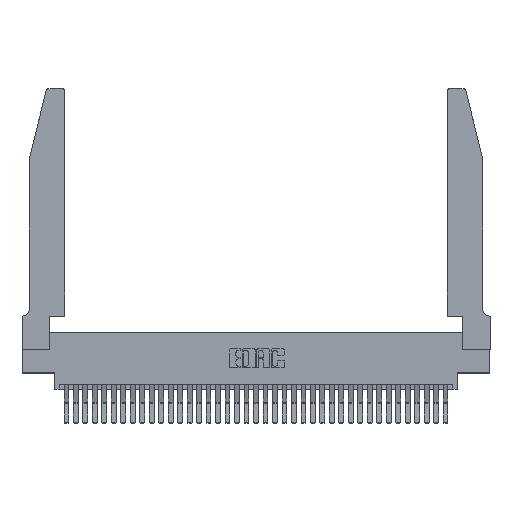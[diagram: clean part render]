
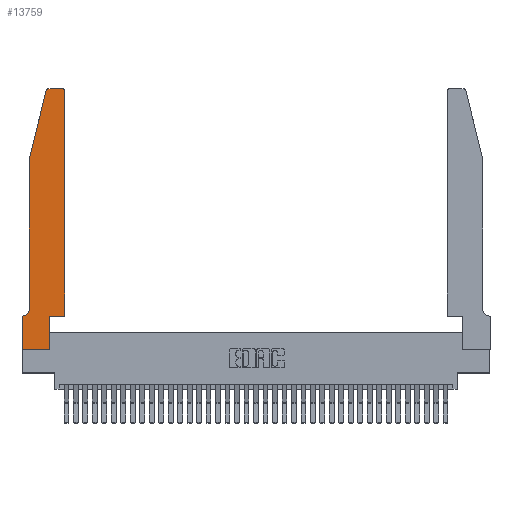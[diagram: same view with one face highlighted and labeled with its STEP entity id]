
A CAD part, top view. The second image highlights one B-rep face of the part: STEP entity #13759.
In plain terms, the highlighted planar face has unit normal (0, 0, 1).
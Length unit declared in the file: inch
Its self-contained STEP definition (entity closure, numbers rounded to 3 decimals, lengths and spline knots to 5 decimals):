
#987 = VERTEX_POINT ( 'NONE', #4956 ) ;
#1030 = EDGE_CURVE ( 'NONE', #20445, #4806, #24378, .T. ) ;
#1146 = DIRECTION ( 'NONE',  ( 0., 1., 0. ) ) ;
#1535 = ORIENTED_EDGE ( 'NONE', *, *, #20701, .T. ) ;
#1690 = CARTESIAN_POINT ( 'NONE',  ( 0.4505, 0.35, 0.37 ) ) ;
#2357 = ORIENTED_EDGE ( 'NONE', *, *, #13382, .T. ) ;
#2497 = CARTESIAN_POINT ( 'NONE',  ( 0.0755, 2., 0.37 ) ) ;
#2549 = CIRCLE ( 'NONE', #15674, 0.03 ) ;
#2687 = VERTEX_POINT ( 'NONE', #11166 ) ;
#3035 = VECTOR ( 'NONE', #26420, 39.37008 ) ;
#3300 = CARTESIAN_POINT ( 'NONE',  ( 0.0055, 0.35, 0.37 ) ) ;
#4227 = ORIENTED_EDGE ( 'NONE', *, *, #7650, .T. ) ;
#4806 = VERTEX_POINT ( 'NONE', #6256 ) ;
#4956 = CARTESIAN_POINT ( 'NONE',  ( 0.0755, 0.42, 0.37 ) ) ;
#5392 = EDGE_CURVE ( 'NONE', #28040, #29373, #31804, .T. ) ;
#5858 = DIRECTION ( 'NONE',  ( 0., 0., 1. ) ) ;
#6211 = VECTOR ( 'NONE', #27358, 39.37008 ) ;
#6256 = CARTESIAN_POINT ( 'NONE',  ( 0.25487, 2.72718, 0.37 ) ) ;
#7337 = VECTOR ( 'NONE', #1146, 39.37008 ) ;
#7357 = CARTESIAN_POINT ( 'NONE',  ( 0., 0., 0.37 ) ) ;
#7650 = EDGE_CURVE ( 'NONE', #9972, #987, #27137, .T. ) ;
#8226 = DIRECTION ( 'NONE',  ( 1., 0., 0. ) ) ;
#8504 = DIRECTION ( 'NONE',  ( 1., 0., 0. ) ) ;
#8624 = CARTESIAN_POINT ( 'NONE',  ( 0., 0.35, 0.37 ) ) ;
#8904 = AXIS2_PLACEMENT_3D ( 'NONE', #16805, #11001, #8226 ) ;
#9054 = VERTEX_POINT ( 'NONE', #22963 ) ;
#9463 = CARTESIAN_POINT ( 'NONE',  ( 0.0755, 2., 0.37 ) ) ;
#9474 = CARTESIAN_POINT ( 'NONE',  ( 0.2865, 0.35, 0.37 ) ) ;
#9972 = VERTEX_POINT ( 'NONE', #9463 ) ;
#10674 = VECTOR ( 'NONE', #16468, 39.37008 ) ;
#11001 = DIRECTION ( 'NONE',  ( 0., 0., 1. ) ) ;
#11166 = CARTESIAN_POINT ( 'NONE',  ( 0.2865, 0., 0.37 ) ) ;
#11451 = DIRECTION ( 'NONE',  ( 0., -1., 0. ) ) ;
#11640 = VECTOR ( 'NONE', #19379, 39.37008 ) ;
#12024 = CARTESIAN_POINT ( 'NONE',  ( 0.4505, 0.35, 0.37 ) ) ;
#13234 = CARTESIAN_POINT ( 'NONE',  ( 0.4205, 2.75, 0.37 ) ) ;
#13375 = VECTOR ( 'NONE', #27454, 39.37008 ) ;
#13382 = EDGE_CURVE ( 'NONE', #24553, #26212, #18349, .T. ) ;
#13530 = ORIENTED_EDGE ( 'NONE', *, *, #33803, .T. ) ;
#13569 = DIRECTION ( 'NONE',  ( -1., 0., 0. ) ) ;
#13759 = ADVANCED_FACE ( 'NONE', ( #29547 ), #22829, .T. ) ;
#13868 = AXIS2_PLACEMENT_3D ( 'NONE', #29996, #19187, #27828 ) ;
#14527 = VECTOR ( 'NONE', #15802, 39.37008 ) ;
#14761 = CARTESIAN_POINT ( 'NONE',  ( 0.4205, 2.72, 0.37 ) ) ;
#15063 = ORIENTED_EDGE ( 'NONE', *, *, #23568, .T. ) ;
#15325 = CARTESIAN_POINT ( 'NONE',  ( 0., 0.35, 0.37 ) ) ;
#15674 = AXIS2_PLACEMENT_3D ( 'NONE', #14761, #26047, #26431 ) ;
#15802 = DIRECTION ( 'NONE',  ( 0., -1., 0. ) ) ;
#16177 = ORIENTED_EDGE ( 'NONE', *, *, #33617, .T. ) ;
#16461 = ORIENTED_EDGE ( 'NONE', *, *, #21335, .T. ) ;
#16468 = DIRECTION ( 'NONE',  ( -0.239, -0.971, 0. ) ) ;
#16805 = CARTESIAN_POINT ( 'NONE',  ( 0.284, 2.72, 0.37 ) ) ;
#17459 = EDGE_CURVE ( 'NONE', #987, #24553, #37148, .T. ) ;
#17504 = CARTESIAN_POINT ( 'NONE',  ( 0.0755, 0.35, 0.37 ) ) ;
#17983 = VECTOR ( 'NONE', #13569, 39.37008 ) ;
#18349 = LINE ( 'NONE', #17504, #3035 ) ;
#18803 = EDGE_CURVE ( 'NONE', #2687, #28040, #29356, .T. ) ;
#19187 = DIRECTION ( 'NONE',  ( 0., 0., -1. ) ) ;
#19379 = DIRECTION ( 'NONE',  ( 1., 0., 0. ) ) ;
#19601 = ORIENTED_EDGE ( 'NONE', *, *, #5392, .T. ) ;
#20445 = VERTEX_POINT ( 'NONE', #29235 ) ;
#20701 = EDGE_CURVE ( 'NONE', #21166, #20445, #33688, .T. ) ;
#21166 = VERTEX_POINT ( 'NONE', #13234 ) ;
#21335 = EDGE_CURVE ( 'NONE', #30478, #2687, #25162, .T. ) ;
#22791 = LINE ( 'NONE', #33625, #10674 ) ;
#22829 = PLANE ( 'NONE',  #34493 ) ;
#22963 = CARTESIAN_POINT ( 'NONE',  ( 0.4505, 2.72, 0.37 ) ) ;
#23144 = VECTOR ( 'NONE', #11451, 39.37008 ) ;
#23568 = EDGE_CURVE ( 'NONE', #9054, #21166, #2549, .T. ) ;
#24378 = CIRCLE ( 'NONE', #8904, 0.03 ) ;
#24553 = VERTEX_POINT ( 'NONE', #3300 ) ;
#25049 = CARTESIAN_POINT ( 'NONE',  ( 0.2605, 2.75, 0.37 ) ) ;
#25162 = LINE ( 'NONE', #28154, #11640 ) ;
#25862 = EDGE_CURVE ( 'NONE', #26212, #30478, #31568, .T. ) ;
#26047 = DIRECTION ( 'NONE',  ( 0., 0., 1. ) ) ;
#26212 = VERTEX_POINT ( 'NONE', #15325 ) ;
#26420 = DIRECTION ( 'NONE',  ( -1., 0., 0. ) ) ;
#26431 = DIRECTION ( 'NONE',  ( 1., 0., 0. ) ) ;
#26809 = EDGE_LOOP ( 'NONE', ( #1535, #36392, #13530, #4227, #30798, #2357, #32501, #16461, #28762, #19601, #16177, #15063 ) ) ;
#27137 = LINE ( 'NONE', #2497, #23144 ) ;
#27358 = DIRECTION ( 'NONE',  ( 1., 0., 0. ) ) ;
#27454 = DIRECTION ( 'NONE',  ( 0., 1., 0. ) ) ;
#27828 = DIRECTION ( 'NONE',  ( -1., 0., 0. ) ) ;
#28040 = VERTEX_POINT ( 'NONE', #36655 ) ;
#28154 = CARTESIAN_POINT ( 'NONE',  ( 0., 0., 0.37 ) ) ;
#28654 = LINE ( 'NONE', #1690, #13375 ) ;
#28762 = ORIENTED_EDGE ( 'NONE', *, *, #18803, .T. ) ;
#29235 = CARTESIAN_POINT ( 'NONE',  ( 0.284, 2.75, 0.37 ) ) ;
#29356 = LINE ( 'NONE', #9474, #7337 ) ;
#29373 = VERTEX_POINT ( 'NONE', #12024 ) ;
#29547 = FACE_OUTER_BOUND ( 'NONE', #26809, .T. ) ;
#29996 = CARTESIAN_POINT ( 'NONE',  ( 0.0055, 0.42, 0.37 ) ) ;
#30478 = VERTEX_POINT ( 'NONE', #32706 ) ;
#30798 = ORIENTED_EDGE ( 'NONE', *, *, #17459, .T. ) ;
#31568 = LINE ( 'NONE', #7357, #14527 ) ;
#31804 = LINE ( 'NONE', #32884, #6211 ) ;
#32501 = ORIENTED_EDGE ( 'NONE', *, *, #25862, .T. ) ;
#32706 = CARTESIAN_POINT ( 'NONE',  ( 0., 0., 0.37 ) ) ;
#32884 = CARTESIAN_POINT ( 'NONE',  ( 0.4505, 0.35, 0.37 ) ) ;
#33617 = EDGE_CURVE ( 'NONE', #29373, #9054, #28654, .T. ) ;
#33625 = CARTESIAN_POINT ( 'NONE',  ( 0.0755, 2., 0.37 ) ) ;
#33688 = LINE ( 'NONE', #25049, #17983 ) ;
#33803 = EDGE_CURVE ( 'NONE', #4806, #9972, #22791, .T. ) ;
#34493 = AXIS2_PLACEMENT_3D ( 'NONE', #8624, #5858, #8504 ) ;
#36392 = ORIENTED_EDGE ( 'NONE', *, *, #1030, .T. ) ;
#36655 = CARTESIAN_POINT ( 'NONE',  ( 0.2865, 0.35, 0.37 ) ) ;
#37148 = CIRCLE ( 'NONE', #13868, 0.07 ) ;
